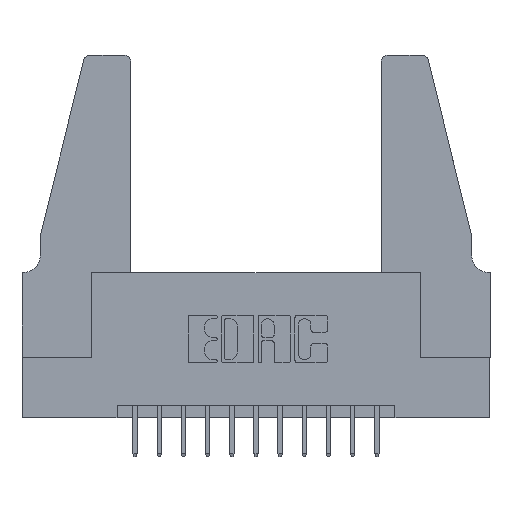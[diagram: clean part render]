
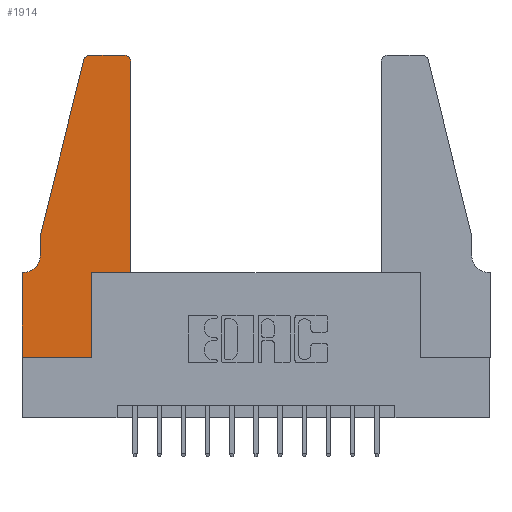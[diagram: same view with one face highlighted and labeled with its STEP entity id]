
A CAD part, top view. The second image highlights one B-rep face of the part: STEP entity #1914.
In plain terms, the highlighted planar face has unit normal (0, 0, 1).
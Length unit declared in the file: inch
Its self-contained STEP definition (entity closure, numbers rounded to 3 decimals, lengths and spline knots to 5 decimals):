
#16 = DIRECTION ( 'NONE',  ( 0., 1., 0. ) ) ;
#88 = VERTEX_POINT ( 'NONE', #1131 ) ;
#114 = LINE ( 'NONE', #5506, #6115 ) ;
#199 = AXIS2_PLACEMENT_3D ( 'NONE', #7222, #11887, #6695 ) ;
#298 = CIRCLE ( 'NONE', #199, 0.03 ) ;
#696 = LINE ( 'NONE', #14124, #9588 ) ;
#988 = CARTESIAN_POINT ( 'NONE',  ( 0.4505, 0.35, 0.37 ) ) ;
#1114 = ORIENTED_EDGE ( 'NONE', *, *, #9534, .T. ) ;
#1131 = CARTESIAN_POINT ( 'NONE',  ( 0.4205, 1.25, 0.37 ) ) ;
#1369 = VERTEX_POINT ( 'NONE', #9985 ) ;
#1412 = ORIENTED_EDGE ( 'NONE', *, *, #3919, .T. ) ;
#1578 = CARTESIAN_POINT ( 'NONE',  ( 0., 0., 0.37 ) ) ;
#1659 = CARTESIAN_POINT ( 'NONE',  ( 0.4505, 1.22, 0.37 ) ) ;
#1888 = VERTEX_POINT ( 'NONE', #10752 ) ;
#1914 = ADVANCED_FACE ( 'NONE', ( #11620 ), #13101, .T. ) ;
#1943 = VECTOR ( 'NONE', #5383, 39.37008 ) ;
#2087 = LINE ( 'NONE', #8239, #6083 ) ;
#2104 = VERTEX_POINT ( 'NONE', #988 ) ;
#2188 = CARTESIAN_POINT ( 'NONE',  ( 0.2865, 0.35, 0.37 ) ) ;
#2247 = ORIENTED_EDGE ( 'NONE', *, *, #7692, .T. ) ;
#2375 = CIRCLE ( 'NONE', #9821, 0.03 ) ;
#3593 = ORIENTED_EDGE ( 'NONE', *, *, #12786, .T. ) ;
#3919 = EDGE_CURVE ( 'NONE', #5007, #12625, #2087, .T. ) ;
#4159 = VERTEX_POINT ( 'NONE', #1659 ) ;
#4174 = LINE ( 'NONE', #14194, #12892 ) ;
#4747 = ORIENTED_EDGE ( 'NONE', *, *, #14382, .T. ) ;
#5007 = VERTEX_POINT ( 'NONE', #7084 ) ;
#5383 = DIRECTION ( 'NONE',  ( 0., -1., 0. ) ) ;
#5399 = DIRECTION ( 'NONE',  ( -1., 0., 0. ) ) ;
#5506 = CARTESIAN_POINT ( 'NONE',  ( 0.4505, 0.35, 0.37 ) ) ;
#5734 = ORIENTED_EDGE ( 'NONE', *, *, #14849, .T. ) ;
#5756 = VERTEX_POINT ( 'NONE', #12463 ) ;
#5779 = VECTOR ( 'NONE', #10194, 39.37008 ) ;
#5822 = VECTOR ( 'NONE', #8791, 39.37008 ) ;
#5870 = EDGE_CURVE ( 'NONE', #4159, #88, #2375, .T. ) ;
#6050 = DIRECTION ( 'NONE',  ( 1., 0., 0. ) ) ;
#6083 = VECTOR ( 'NONE', #13920, 39.37008 ) ;
#6115 = VECTOR ( 'NONE', #8957, 39.37008 ) ;
#6165 = DIRECTION ( 'NONE',  ( 0., -1., 0. ) ) ;
#6695 = DIRECTION ( 'NONE',  ( 1., 0., 0. ) ) ;
#6845 = EDGE_CURVE ( 'NONE', #88, #5756, #14706, .T. ) ;
#6868 = LINE ( 'NONE', #7952, #5779 ) ;
#7084 = CARTESIAN_POINT ( 'NONE',  ( 0.0055, 0.35, 0.37 ) ) ;
#7222 = CARTESIAN_POINT ( 'NONE',  ( 0.284, 1.22, 0.37 ) ) ;
#7360 = EDGE_CURVE ( 'NONE', #14835, #1888, #696, .T. ) ;
#7449 = VERTEX_POINT ( 'NONE', #1578 ) ;
#7692 = EDGE_CURVE ( 'NONE', #11810, #2104, #6868, .T. ) ;
#7856 = ORIENTED_EDGE ( 'NONE', *, *, #11859, .T. ) ;
#7952 = CARTESIAN_POINT ( 'NONE',  ( 0.4505, 0.35, 0.37 ) ) ;
#7998 = EDGE_LOOP ( 'NONE', ( #12895, #12458, #5734, #12088, #4747, #1412, #13795, #7856, #3593, #2247, #1114, #8879 ) ) ;
#8040 = DIRECTION ( 'NONE',  ( 1., 0., 0. ) ) ;
#8239 = CARTESIAN_POINT ( 'NONE',  ( 0.0755, 0.35, 0.37 ) ) ;
#8791 = DIRECTION ( 'NONE',  ( -1., 0., 0. ) ) ;
#8849 = EDGE_CURVE ( 'NONE', #5756, #1369, #298, .T. ) ;
#8879 = ORIENTED_EDGE ( 'NONE', *, *, #5870, .T. ) ;
#8957 = DIRECTION ( 'NONE',  ( 0., 1., 0. ) ) ;
#8977 = LINE ( 'NONE', #10225, #11689 ) ;
#9205 = EDGE_CURVE ( 'NONE', #12625, #7449, #10463, .T. ) ;
#9534 = EDGE_CURVE ( 'NONE', #2104, #4159, #114, .T. ) ;
#9588 = VECTOR ( 'NONE', #6165, 39.37008 ) ;
#9821 = AXIS2_PLACEMENT_3D ( 'NONE', #11836, #14150, #6050 ) ;
#9985 = CARTESIAN_POINT ( 'NONE',  ( 0.25487, 1.22718, 0.37 ) ) ;
#10194 = DIRECTION ( 'NONE',  ( 1., 0., 0. ) ) ;
#10225 = CARTESIAN_POINT ( 'NONE',  ( 0., 0., 0.37 ) ) ;
#10463 = LINE ( 'NONE', #11314, #1943 ) ;
#10752 = CARTESIAN_POINT ( 'NONE',  ( 0.0755, 0.42, 0.37 ) ) ;
#11314 = CARTESIAN_POINT ( 'NONE',  ( 0., 0., 0.37 ) ) ;
#11523 = VERTEX_POINT ( 'NONE', #12909 ) ;
#11620 = FACE_OUTER_BOUND ( 'NONE', #7998, .T. ) ;
#11689 = VECTOR ( 'NONE', #8040, 39.37008 ) ;
#11751 = DIRECTION ( 'NONE',  ( 0., 0., 1. ) ) ;
#11810 = VERTEX_POINT ( 'NONE', #12332 ) ;
#11831 = DIRECTION ( 'NONE',  ( -0.239, -0.971, 0. ) ) ;
#11836 = CARTESIAN_POINT ( 'NONE',  ( 0.4205, 1.22, 0.37 ) ) ;
#11859 = EDGE_CURVE ( 'NONE', #7449, #11523, #8977, .T. ) ;
#11882 = CARTESIAN_POINT ( 'NONE',  ( 0.0755, 0.5, 0.37 ) ) ;
#11887 = DIRECTION ( 'NONE',  ( 0., 0., 1. ) ) ;
#12039 = VECTOR ( 'NONE', #16, 39.37008 ) ;
#12088 = ORIENTED_EDGE ( 'NONE', *, *, #7360, .T. ) ;
#12332 = CARTESIAN_POINT ( 'NONE',  ( 0.2865, 0.35, 0.37 ) ) ;
#12458 = ORIENTED_EDGE ( 'NONE', *, *, #8849, .T. ) ;
#12463 = CARTESIAN_POINT ( 'NONE',  ( 0.284, 1.25, 0.37 ) ) ;
#12625 = VERTEX_POINT ( 'NONE', #12768 ) ;
#12768 = CARTESIAN_POINT ( 'NONE',  ( 0., 0.35, 0.37 ) ) ;
#12786 = EDGE_CURVE ( 'NONE', #11523, #11810, #13297, .T. ) ;
#12840 = AXIS2_PLACEMENT_3D ( 'NONE', #14624, #14671, #5399 ) ;
#12892 = VECTOR ( 'NONE', #11831, 39.37008 ) ;
#12895 = ORIENTED_EDGE ( 'NONE', *, *, #6845, .T. ) ;
#12909 = CARTESIAN_POINT ( 'NONE',  ( 0.2865, 0., 0.37 ) ) ;
#13101 = PLANE ( 'NONE',  #14647 ) ;
#13297 = LINE ( 'NONE', #2188, #12039 ) ;
#13795 = ORIENTED_EDGE ( 'NONE', *, *, #9205, .T. ) ;
#13920 = DIRECTION ( 'NONE',  ( -1., 0., 0. ) ) ;
#14062 = DIRECTION ( 'NONE',  ( 1., 0., 0. ) ) ;
#14111 = CARTESIAN_POINT ( 'NONE',  ( 0., 0.35, 0.37 ) ) ;
#14124 = CARTESIAN_POINT ( 'NONE',  ( 0.0755, 0.5, 0.37 ) ) ;
#14150 = DIRECTION ( 'NONE',  ( 0., 0., 1. ) ) ;
#14194 = CARTESIAN_POINT ( 'NONE',  ( 0.0755, 0.5, 0.37 ) ) ;
#14323 = CIRCLE ( 'NONE', #12840, 0.07 ) ;
#14382 = EDGE_CURVE ( 'NONE', #1888, #5007, #14323, .T. ) ;
#14491 = CARTESIAN_POINT ( 'NONE',  ( 0.2605, 1.25, 0.37 ) ) ;
#14624 = CARTESIAN_POINT ( 'NONE',  ( 0.0055, 0.42, 0.37 ) ) ;
#14647 = AXIS2_PLACEMENT_3D ( 'NONE', #14111, #11751, #14062 ) ;
#14671 = DIRECTION ( 'NONE',  ( 0., 0., -1. ) ) ;
#14706 = LINE ( 'NONE', #14491, #5822 ) ;
#14835 = VERTEX_POINT ( 'NONE', #11882 ) ;
#14849 = EDGE_CURVE ( 'NONE', #1369, #14835, #4174, .T. ) ;
